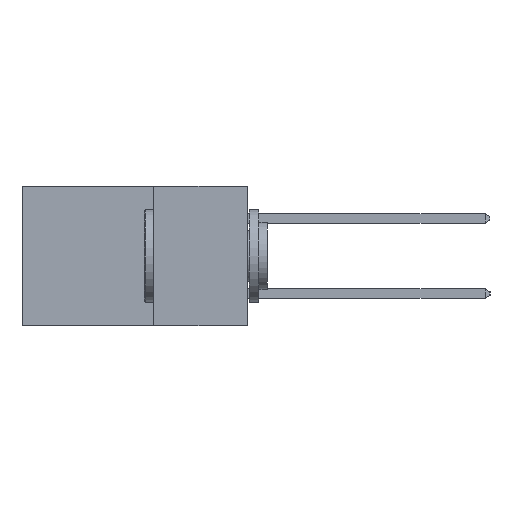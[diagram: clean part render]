
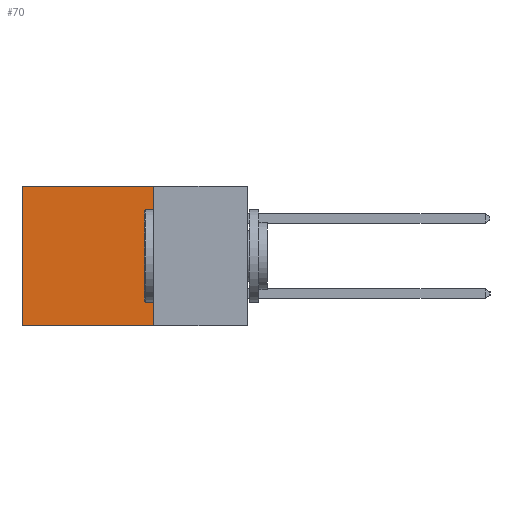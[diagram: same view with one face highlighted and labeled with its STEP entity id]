
A CAD part, left-side view. The second image highlights one B-rep face of the part: STEP entity #70.
In plain terms, the highlighted planar face has unit normal (-1, 0, 0).
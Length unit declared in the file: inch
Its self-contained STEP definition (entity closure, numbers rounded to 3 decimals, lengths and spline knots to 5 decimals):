
#14 = CARTESIAN_POINT ( 'NONE',  ( 0.2615, 0.25, 0. ) ) ;
#70 = ADVANCED_FACE ( 'NONE', ( #5474 ), #6234, .F. ) ;
#910 = CARTESIAN_POINT ( 'NONE',  ( 0.2615, 0.25, -0.37 ) ) ;
#1205 = LINE ( 'NONE', #14, #11061 ) ;
#1444 = VECTOR ( 'NONE', #11184, 39.37008 ) ;
#2392 = CARTESIAN_POINT ( 'NONE',  ( 0.2615, 0.25, 0. ) ) ;
#2738 = CARTESIAN_POINT ( 'NONE',  ( 0.2615, 0.25, -0.37 ) ) ;
#3141 = DIRECTION ( 'NONE',  ( 0., 1., 0. ) ) ;
#3249 = CARTESIAN_POINT ( 'NONE',  ( 0.2615, 0.25, -0.37 ) ) ;
#3642 = VERTEX_POINT ( 'NONE', #3249 ) ;
#3925 = VECTOR ( 'NONE', #9980, 39.37008 ) ;
#4223 = VERTEX_POINT ( 'NONE', #6195 ) ;
#4911 = ORIENTED_EDGE ( 'NONE', *, *, #9104, .F. ) ;
#5348 = ORIENTED_EDGE ( 'NONE', *, *, #15058, .F. ) ;
#5474 = FACE_OUTER_BOUND ( 'NONE', #8945, .T. ) ;
#6195 = CARTESIAN_POINT ( 'NONE',  ( 0.2615, 0.6, -0.37 ) ) ;
#6215 = CARTESIAN_POINT ( 'NONE',  ( 0.2615, 0.25, -0.37 ) ) ;
#6234 = PLANE ( 'NONE',  #12075 ) ;
#7798 = EDGE_CURVE ( 'NONE', #10907, #9661, #1205, .T. ) ;
#8448 = VECTOR ( 'NONE', #3141, 39.37008 ) ;
#8460 = DIRECTION ( 'NONE',  ( 0., 1., 0. ) ) ;
#8945 = EDGE_LOOP ( 'NONE', ( #11299, #4911, #5348, #9133 ) ) ;
#9104 = EDGE_CURVE ( 'NONE', #3642, #4223, #11808, .T. ) ;
#9133 = ORIENTED_EDGE ( 'NONE', *, *, #7798, .T. ) ;
#9661 = VERTEX_POINT ( 'NONE', #12701 ) ;
#9802 = DIRECTION ( 'NONE',  ( 1., 0., 0. ) ) ;
#9980 = DIRECTION ( 'NONE',  ( 0., 0., -1. ) ) ;
#10026 = CARTESIAN_POINT ( 'NONE',  ( 0.2615, 0.6, -0.37 ) ) ;
#10740 = LINE ( 'NONE', #10026, #3925 ) ;
#10907 = VERTEX_POINT ( 'NONE', #2392 ) ;
#11061 = VECTOR ( 'NONE', #8460, 39.37008 ) ;
#11184 = DIRECTION ( 'NONE',  ( 0., 0., -1. ) ) ;
#11299 = ORIENTED_EDGE ( 'NONE', *, *, #13341, .T. ) ;
#11808 = LINE ( 'NONE', #2738, #8448 ) ;
#12075 = AXIS2_PLACEMENT_3D ( 'NONE', #6215, #9802, #13381 ) ;
#12076 = LINE ( 'NONE', #910, #1444 ) ;
#12701 = CARTESIAN_POINT ( 'NONE',  ( 0.2615, 0.6, 0. ) ) ;
#13341 = EDGE_CURVE ( 'NONE', #9661, #4223, #10740, .T. ) ;
#13381 = DIRECTION ( 'NONE',  ( 0., 0., -1. ) ) ;
#15058 = EDGE_CURVE ( 'NONE', #10907, #3642, #12076, .T. ) ;
